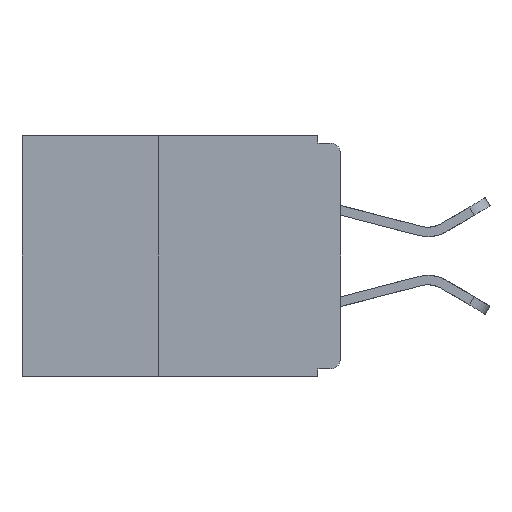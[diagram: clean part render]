
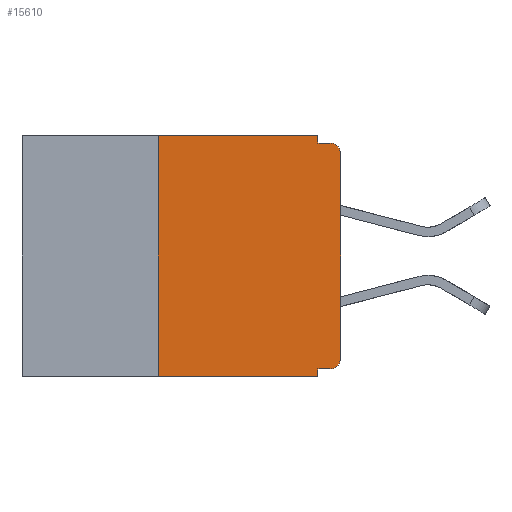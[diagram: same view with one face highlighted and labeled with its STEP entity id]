
A CAD part, left-side view. The second image highlights one B-rep face of the part: STEP entity #15610.
In plain terms, the highlighted planar face has unit normal (-1, 0, 0).
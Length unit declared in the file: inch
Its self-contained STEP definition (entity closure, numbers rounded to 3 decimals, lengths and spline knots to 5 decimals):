
#486 = ORIENTED_EDGE ( 'NONE', *, *, #6429, .T. ) ;
#805 = ORIENTED_EDGE ( 'NONE', *, *, #3416, .F. ) ;
#1564 = VECTOR ( 'NONE', #20268, 39.37008 ) ;
#1583 = CARTESIAN_POINT ( 'NONE',  ( 0., 0.031, -0.32 ) ) ;
#2112 = LINE ( 'NONE', #16985, #23342 ) ;
#2118 = EDGE_CURVE ( 'NONE', #22552, #22979, #14493, .T. ) ;
#2233 = CARTESIAN_POINT ( 'NONE',  ( 0., 0.25, -0.33 ) ) ;
#2389 = VERTEX_POINT ( 'NONE', #21617 ) ;
#2557 = LINE ( 'NONE', #13548, #23747 ) ;
#2920 = VERTEX_POINT ( 'NONE', #20205 ) ;
#3266 = AXIS2_PLACEMENT_3D ( 'NONE', #22568, #10421, #24568 ) ;
#3356 = CARTESIAN_POINT ( 'NONE',  ( 0., 0., -0.32 ) ) ;
#3416 = EDGE_CURVE ( 'NONE', #2389, #18186, #2112, .T. ) ;
#3464 = AXIS2_PLACEMENT_3D ( 'NONE', #8005, #22274, #10112 ) ;
#3792 = VECTOR ( 'NONE', #5525, 39.37008 ) ;
#4186 = CIRCLE ( 'NONE', #3464, 0.015 ) ;
#4858 = DIRECTION ( 'NONE',  ( 0., -1., 0. ) ) ;
#4872 = ORIENTED_EDGE ( 'NONE', *, *, #15985, .F. ) ;
#4964 = EDGE_CURVE ( 'NONE', #18186, #26290, #10587, .T. ) ;
#5525 = DIRECTION ( 'NONE',  ( 0., 1., 0. ) ) ;
#6429 = EDGE_CURVE ( 'NONE', #6645, #2920, #18121, .T. ) ;
#6645 = VERTEX_POINT ( 'NONE', #20956 ) ;
#7537 = VERTEX_POINT ( 'NONE', #11479 ) ;
#7714 = CARTESIAN_POINT ( 'NONE',  ( 0., 0.031, -0.33 ) ) ;
#7751 = EDGE_CURVE ( 'NONE', #14019, #6645, #4186, .T. ) ;
#8005 = CARTESIAN_POINT ( 'NONE',  ( 0., 0.015, -0.305 ) ) ;
#8122 = LINE ( 'NONE', #8739, #18375 ) ;
#8259 = LINE ( 'NONE', #17091, #23856 ) ;
#8739 = CARTESIAN_POINT ( 'NONE',  ( 0., 0., -0.01 ) ) ;
#9479 = CARTESIAN_POINT ( 'NONE',  ( 0., 0.031, 0. ) ) ;
#9485 = DIRECTION ( 'NONE',  ( 0., 0., -1. ) ) ;
#9765 = CARTESIAN_POINT ( 'NONE',  ( 0., 0.015, -0.025 ) ) ;
#9924 = VECTOR ( 'NONE', #9485, 39.37008 ) ;
#10112 = DIRECTION ( 'NONE',  ( 0., 0., -1. ) ) ;
#10330 = PLANE ( 'NONE',  #3266 ) ;
#10409 = VERTEX_POINT ( 'NONE', #2233 ) ;
#10421 = DIRECTION ( 'NONE',  ( 1., 0., 0. ) ) ;
#10587 = LINE ( 'NONE', #9479, #9924 ) ;
#10702 = ORIENTED_EDGE ( 'NONE', *, *, #16415, .F. ) ;
#11340 = ORIENTED_EDGE ( 'NONE', *, *, #4964, .F. ) ;
#11479 = CARTESIAN_POINT ( 'NONE',  ( 0., 0.015, -0.01 ) ) ;
#11860 = DIRECTION ( 'NONE',  ( 0., 0., -1. ) ) ;
#12467 = AXIS2_PLACEMENT_3D ( 'NONE', #9765, #23953, #11860 ) ;
#12750 = CARTESIAN_POINT ( 'NONE',  ( 0., 0.015, -0.32 ) ) ;
#12891 = DIRECTION ( 'NONE',  ( 0., -1., 0. ) ) ;
#13548 = CARTESIAN_POINT ( 'NONE',  ( 0., 0.25, -0.33 ) ) ;
#13880 = VECTOR ( 'NONE', #16177, 39.37008 ) ;
#14019 = VERTEX_POINT ( 'NONE', #12750 ) ;
#14493 = LINE ( 'NONE', #16173, #13880 ) ;
#15562 = DIRECTION ( 'NONE',  ( 0., 0., 1. ) ) ;
#15610 = ADVANCED_FACE ( 'NONE', ( #18863 ), #10330, .F. ) ;
#15830 = EDGE_CURVE ( 'NONE', #10409, #22979, #8259, .T. ) ;
#15835 = ORIENTED_EDGE ( 'NONE', *, *, #15830, .T. ) ;
#15985 = EDGE_CURVE ( 'NONE', #10409, #2389, #2557, .T. ) ;
#16037 = EDGE_LOOP ( 'NONE', ( #486, #22430, #10702, #11340, #805, #4872, #15835, #19703, #21903, #21016 ) ) ;
#16173 = CARTESIAN_POINT ( 'NONE',  ( 0., 0.031, -0.33 ) ) ;
#16177 = DIRECTION ( 'NONE',  ( 0., 0., -1. ) ) ;
#16415 = EDGE_CURVE ( 'NONE', #26290, #7537, #8122, .T. ) ;
#16985 = CARTESIAN_POINT ( 'NONE',  ( 0., 0.437, 0. ) ) ;
#17091 = CARTESIAN_POINT ( 'NONE',  ( 0., 0.437, -0.33 ) ) ;
#17206 = EDGE_CURVE ( 'NONE', #14019, #22552, #20900, .T. ) ;
#18121 = LINE ( 'NONE', #26210, #1564 ) ;
#18186 = VERTEX_POINT ( 'NONE', #24019 ) ;
#18375 = VECTOR ( 'NONE', #12891, 39.37008 ) ;
#18439 = DIRECTION ( 'NONE',  ( 0., -1., 0. ) ) ;
#18494 = CIRCLE ( 'NONE', #12467, 0.015 ) ;
#18863 = FACE_OUTER_BOUND ( 'NONE', #16037, .T. ) ;
#19703 = ORIENTED_EDGE ( 'NONE', *, *, #2118, .F. ) ;
#20205 = CARTESIAN_POINT ( 'NONE',  ( 0., 0., -0.025 ) ) ;
#20268 = DIRECTION ( 'NONE',  ( 0., 0., 1. ) ) ;
#20314 = CARTESIAN_POINT ( 'NONE',  ( 0., 0.031, -0.01 ) ) ;
#20900 = LINE ( 'NONE', #3356, #3792 ) ;
#20956 = CARTESIAN_POINT ( 'NONE',  ( 0., 0., -0.305 ) ) ;
#21016 = ORIENTED_EDGE ( 'NONE', *, *, #7751, .T. ) ;
#21617 = CARTESIAN_POINT ( 'NONE',  ( 0., 0.25, 0. ) ) ;
#21903 = ORIENTED_EDGE ( 'NONE', *, *, #17206, .F. ) ;
#22274 = DIRECTION ( 'NONE',  ( -1., 0., 0. ) ) ;
#22430 = ORIENTED_EDGE ( 'NONE', *, *, #24733, .T. ) ;
#22552 = VERTEX_POINT ( 'NONE', #1583 ) ;
#22568 = CARTESIAN_POINT ( 'NONE',  ( 0., 0.437, 0. ) ) ;
#22979 = VERTEX_POINT ( 'NONE', #7714 ) ;
#23342 = VECTOR ( 'NONE', #18439, 39.37008 ) ;
#23747 = VECTOR ( 'NONE', #15562, 39.37008 ) ;
#23856 = VECTOR ( 'NONE', #4858, 39.37008 ) ;
#23953 = DIRECTION ( 'NONE',  ( -1., 0., 0. ) ) ;
#24019 = CARTESIAN_POINT ( 'NONE',  ( 0., 0.031, 0. ) ) ;
#24568 = DIRECTION ( 'NONE',  ( 0., 0., -1. ) ) ;
#24733 = EDGE_CURVE ( 'NONE', #2920, #7537, #18494, .T. ) ;
#26210 = CARTESIAN_POINT ( 'NONE',  ( 0., 0., 0. ) ) ;
#26290 = VERTEX_POINT ( 'NONE', #20314 ) ;
